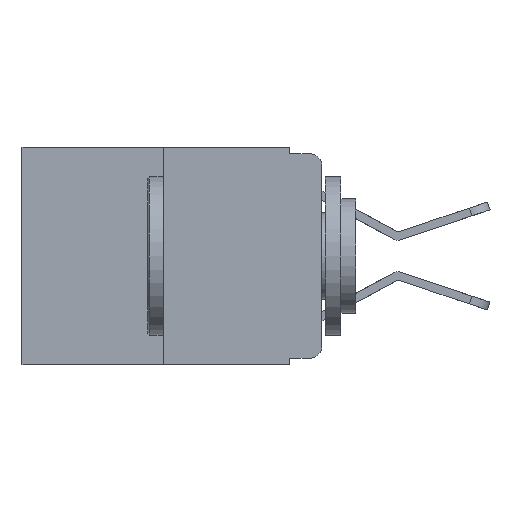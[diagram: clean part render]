
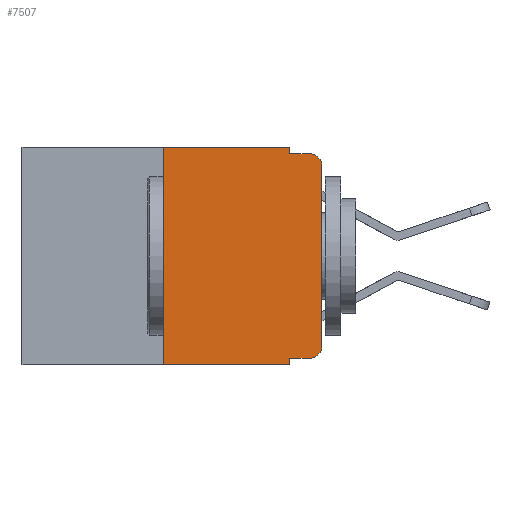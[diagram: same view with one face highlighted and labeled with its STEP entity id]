
A CAD part, left-side view. The second image highlights one B-rep face of the part: STEP entity #7507.
In plain terms, the highlighted planar face has unit normal (-1, 0, 0).
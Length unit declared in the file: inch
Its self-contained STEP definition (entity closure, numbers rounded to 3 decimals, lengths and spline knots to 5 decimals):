
#252 = DIRECTION ( 'NONE',  ( -1., 0., 0. ) ) ;
#767 = CIRCLE ( 'NONE', #8325, 0.02 ) ;
#817 = VECTOR ( 'NONE', #5495, 39.37008 ) ;
#832 = CARTESIAN_POINT ( 'NONE',  ( 0., 0., 0. ) ) ;
#1162 = CIRCLE ( 'NONE', #6014, 0.02 ) ;
#1221 = CARTESIAN_POINT ( 'NONE',  ( 0., 0.051, -0.333 ) ) ;
#1429 = EDGE_CURVE ( 'NONE', #5207, #8349, #1162, .T. ) ;
#1686 = LINE ( 'NONE', #7546, #3700 ) ;
#1892 = VERTEX_POINT ( 'NONE', #4543 ) ;
#1988 = CARTESIAN_POINT ( 'NONE',  ( 0., 0.473, 0. ) ) ;
#1992 = VERTEX_POINT ( 'NONE', #11387 ) ;
#2003 = LINE ( 'NONE', #7000, #4013 ) ;
#2023 = CARTESIAN_POINT ( 'NONE',  ( 0., 0.051, 0. ) ) ;
#2143 = ORIENTED_EDGE ( 'NONE', *, *, #7346, .F. ) ;
#2323 = EDGE_CURVE ( 'NONE', #7675, #9204, #8607, .T. ) ;
#2578 = EDGE_CURVE ( 'NONE', #10810, #1992, #8454, .T. ) ;
#2623 = ORIENTED_EDGE ( 'NONE', *, *, #10086, .F. ) ;
#2689 = LINE ( 'NONE', #10673, #12310 ) ;
#2975 = DIRECTION ( 'NONE',  ( 0., 0., -1. ) ) ;
#3018 = DIRECTION ( 'NONE',  ( 0., 0., -1. ) ) ;
#3315 = ORIENTED_EDGE ( 'NONE', *, *, #2323, .F. ) ;
#3320 = VECTOR ( 'NONE', #4749, 39.37008 ) ;
#3427 = LINE ( 'NONE', #12129, #817 ) ;
#3666 = DIRECTION ( 'NONE',  ( 0., 0., -1. ) ) ;
#3700 = VECTOR ( 'NONE', #3666, 39.37008 ) ;
#3911 = ORIENTED_EDGE ( 'NONE', *, *, #10235, .T. ) ;
#4013 = VECTOR ( 'NONE', #7954, 39.37008 ) ;
#4146 = EDGE_CURVE ( 'NONE', #10810, #11217, #2003, .T. ) ;
#4199 = EDGE_CURVE ( 'NONE', #5518, #1892, #767, .T. ) ;
#4303 = CARTESIAN_POINT ( 'NONE',  ( 0., 0., -0.313 ) ) ;
#4346 = VERTEX_POINT ( 'NONE', #9191 ) ;
#4469 = ORIENTED_EDGE ( 'NONE', *, *, #1429, .T. ) ;
#4543 = CARTESIAN_POINT ( 'NONE',  ( 0., 0.02, -0.01 ) ) ;
#4749 = DIRECTION ( 'NONE',  ( 0., 0., 1. ) ) ;
#5017 = ORIENTED_EDGE ( 'NONE', *, *, #2578, .F. ) ;
#5123 = EDGE_LOOP ( 'NONE', ( #7473, #6391, #2623, #3315, #8639, #5017, #5406, #2143, #3911, #4469 ) ) ;
#5207 = VERTEX_POINT ( 'NONE', #9461 ) ;
#5406 = ORIENTED_EDGE ( 'NONE', *, *, #4146, .T. ) ;
#5495 = DIRECTION ( 'NONE',  ( 0., -1., 0. ) ) ;
#5518 = VERTEX_POINT ( 'NONE', #6115 ) ;
#6014 = AXIS2_PLACEMENT_3D ( 'NONE', #9842, #7422, #8474 ) ;
#6056 = VECTOR ( 'NONE', #3018, 39.37008 ) ;
#6115 = CARTESIAN_POINT ( 'NONE',  ( 0., 0., -0.03 ) ) ;
#6128 = DIRECTION ( 'NONE',  ( 0., -1., 0. ) ) ;
#6146 = CARTESIAN_POINT ( 'NONE',  ( 0., 0.02, -0.03 ) ) ;
#6196 = VECTOR ( 'NONE', #6521, 39.37008 ) ;
#6197 = CARTESIAN_POINT ( 'NONE',  ( 0., 0.051, 0. ) ) ;
#6391 = ORIENTED_EDGE ( 'NONE', *, *, #4199, .T. ) ;
#6521 = DIRECTION ( 'NONE',  ( 0., 0., 1. ) ) ;
#6783 = FACE_OUTER_BOUND ( 'NONE', #5123, .T. ) ;
#6786 = CARTESIAN_POINT ( 'NONE',  ( 0., 0.051, -0.343 ) ) ;
#7000 = CARTESIAN_POINT ( 'NONE',  ( 0., 0.473, -0.343 ) ) ;
#7110 = DIRECTION ( 'NONE',  ( 0., 0., -1. ) ) ;
#7302 = CARTESIAN_POINT ( 'NONE',  ( 0., 0.25, 0. ) ) ;
#7346 = EDGE_CURVE ( 'NONE', #4346, #11217, #1686, .T. ) ;
#7422 = DIRECTION ( 'NONE',  ( -1., 0., 0. ) ) ;
#7473 = ORIENTED_EDGE ( 'NONE', *, *, #9993, .T. ) ;
#7507 = ADVANCED_FACE ( 'NONE', ( #6783 ), #7839, .F. ) ;
#7546 = CARTESIAN_POINT ( 'NONE',  ( 0., 0.051, 0. ) ) ;
#7675 = VERTEX_POINT ( 'NONE', #6197 ) ;
#7839 = PLANE ( 'NONE',  #8593 ) ;
#7954 = DIRECTION ( 'NONE',  ( 0., -1., 0. ) ) ;
#8039 = LINE ( 'NONE', #1221, #10292 ) ;
#8325 = AXIS2_PLACEMENT_3D ( 'NONE', #6146, #252, #7110 ) ;
#8349 = VERTEX_POINT ( 'NONE', #4303 ) ;
#8454 = LINE ( 'NONE', #7302, #6196 ) ;
#8474 = DIRECTION ( 'NONE',  ( 0., 0., -1. ) ) ;
#8593 = AXIS2_PLACEMENT_3D ( 'NONE', #1988, #8807, #2975 ) ;
#8607 = LINE ( 'NONE', #2023, #6056 ) ;
#8639 = ORIENTED_EDGE ( 'NONE', *, *, #12126, .F. ) ;
#8807 = DIRECTION ( 'NONE',  ( 1., 0., 0. ) ) ;
#9191 = CARTESIAN_POINT ( 'NONE',  ( 0., 0.051, -0.333 ) ) ;
#9204 = VERTEX_POINT ( 'NONE', #11935 ) ;
#9461 = CARTESIAN_POINT ( 'NONE',  ( 0., 0.02, -0.333 ) ) ;
#9842 = CARTESIAN_POINT ( 'NONE',  ( 0., 0.02, -0.313 ) ) ;
#9993 = EDGE_CURVE ( 'NONE', #8349, #5518, #11009, .T. ) ;
#10086 = EDGE_CURVE ( 'NONE', #9204, #1892, #2689, .T. ) ;
#10235 = EDGE_CURVE ( 'NONE', #4346, #5207, #8039, .T. ) ;
#10292 = VECTOR ( 'NONE', #6128, 39.37008 ) ;
#10673 = CARTESIAN_POINT ( 'NONE',  ( 0., 0.051, -0.01 ) ) ;
#10810 = VERTEX_POINT ( 'NONE', #11790 ) ;
#11009 = LINE ( 'NONE', #832, #3320 ) ;
#11217 = VERTEX_POINT ( 'NONE', #6786 ) ;
#11387 = CARTESIAN_POINT ( 'NONE',  ( 0., 0.25, 0. ) ) ;
#11602 = DIRECTION ( 'NONE',  ( 0., -1., 0. ) ) ;
#11790 = CARTESIAN_POINT ( 'NONE',  ( 0., 0.25, -0.343 ) ) ;
#11935 = CARTESIAN_POINT ( 'NONE',  ( 0., 0.051, -0.01 ) ) ;
#12126 = EDGE_CURVE ( 'NONE', #1992, #7675, #3427, .T. ) ;
#12129 = CARTESIAN_POINT ( 'NONE',  ( 0., 0.473, 0. ) ) ;
#12310 = VECTOR ( 'NONE', #11602, 39.37008 ) ;
